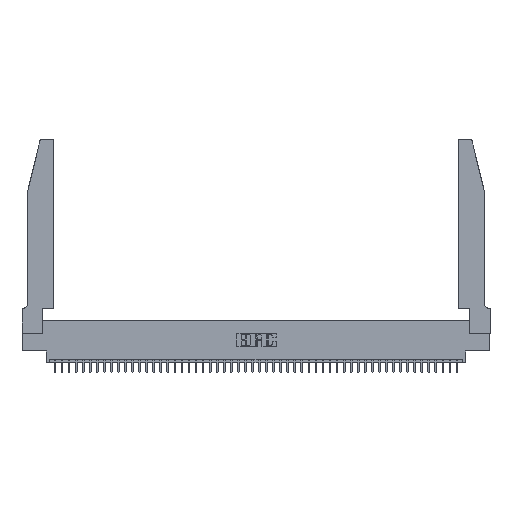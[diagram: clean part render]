
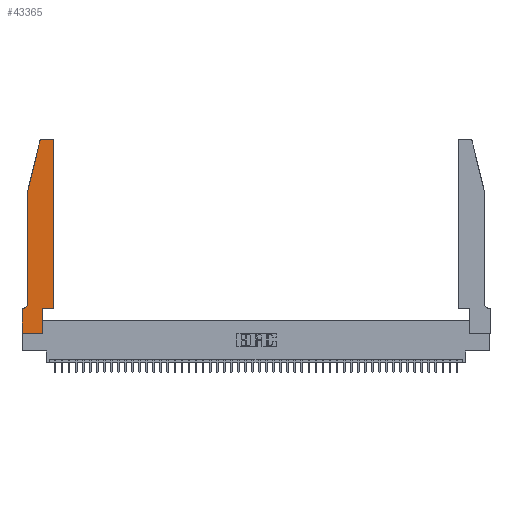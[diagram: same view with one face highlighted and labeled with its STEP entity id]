
A CAD part, top view. The second image highlights one B-rep face of the part: STEP entity #43365.
In plain terms, the highlighted planar face has unit normal (0, 0, 1).
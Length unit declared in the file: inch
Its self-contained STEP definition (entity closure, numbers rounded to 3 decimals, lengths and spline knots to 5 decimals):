
#545 = EDGE_CURVE ( 'NONE', #10601, #28192, #1196, .T. ) ;
#550 = VECTOR ( 'NONE', #3537, 39.37008 ) ;
#1196 = LINE ( 'NONE', #43739, #39708 ) ;
#1553 = VECTOR ( 'NONE', #6246, 39.37008 ) ;
#1555 = CARTESIAN_POINT ( 'NONE',  ( 0.2865, 0.35, 0.37 ) ) ;
#2090 = CARTESIAN_POINT ( 'NONE',  ( 0.2605, 2.75, 0.37 ) ) ;
#2269 = CIRCLE ( 'NONE', #10251, 0.03 ) ;
#2716 = AXIS2_PLACEMENT_3D ( 'NONE', #20783, #46829, #24542 ) ;
#2834 = CIRCLE ( 'NONE', #2716, 0.07 ) ;
#3537 = DIRECTION ( 'NONE',  ( 0., -1., 0. ) ) ;
#4672 = CARTESIAN_POINT ( 'NONE',  ( 0.0755, 0.35, 0.37 ) ) ;
#5462 = CARTESIAN_POINT ( 'NONE',  ( 0.0055, 0.35, 0.37 ) ) ;
#6246 = DIRECTION ( 'NONE',  ( 1., 0., 0. ) ) ;
#6683 = DIRECTION ( 'NONE',  ( 0., 0., 1. ) ) ;
#7171 = VECTOR ( 'NONE', #11006, 39.37008 ) ;
#8366 = VECTOR ( 'NONE', #9087, 39.37008 ) ;
#8771 = CARTESIAN_POINT ( 'NONE',  ( 0., 0.35, 0.37 ) ) ;
#8933 = CARTESIAN_POINT ( 'NONE',  ( 0.4505, 0.35, 0.37 ) ) ;
#9087 = DIRECTION ( 'NONE',  ( 0., 1., 0. ) ) ;
#9230 = VECTOR ( 'NONE', #24424, 39.37008 ) ;
#10251 = AXIS2_PLACEMENT_3D ( 'NONE', #28985, #6683, #32735 ) ;
#10310 = ORIENTED_EDGE ( 'NONE', *, *, #35866, .T. ) ;
#10337 = EDGE_LOOP ( 'NONE', ( #19519, #45235, #38002, #11027, #36350, #38988, #10310, #10574, #17658, #32203, #12888, #32692 ) ) ;
#10574 = ORIENTED_EDGE ( 'NONE', *, *, #18602, .T. ) ;
#10601 = VERTEX_POINT ( 'NONE', #22749 ) ;
#10939 = EDGE_CURVE ( 'NONE', #19008, #40300, #19494, .T. ) ;
#11006 = DIRECTION ( 'NONE',  ( 0., 1., 0. ) ) ;
#11027 = ORIENTED_EDGE ( 'NONE', *, *, #545, .T. ) ;
#12274 = CARTESIAN_POINT ( 'NONE',  ( 0.4505, 2.72, 0.37 ) ) ;
#12522 = DIRECTION ( 'NONE',  ( 1., 0., 0. ) ) ;
#12567 = EDGE_CURVE ( 'NONE', #17947, #24083, #40912, .T. ) ;
#12620 = LINE ( 'NONE', #20073, #31216 ) ;
#12888 = ORIENTED_EDGE ( 'NONE', *, *, #21205, .T. ) ;
#13624 = DIRECTION ( 'NONE',  ( 0., 0., 1. ) ) ;
#14572 = EDGE_CURVE ( 'NONE', #28192, #17947, #2834, .T. ) ;
#14744 = CARTESIAN_POINT ( 'NONE',  ( 0.4505, 0.35, 0.37 ) ) ;
#14824 = CARTESIAN_POINT ( 'NONE',  ( 0.4505, 0.35, 0.37 ) ) ;
#15294 = VERTEX_POINT ( 'NONE', #36340 ) ;
#15814 = EDGE_CURVE ( 'NONE', #40300, #15294, #27862, .T. ) ;
#15906 = DIRECTION ( 'NONE',  ( -1., 0., 0. ) ) ;
#16065 = PLANE ( 'NONE',  #46668 ) ;
#16336 = DIRECTION ( 'NONE',  ( -0.239, -0.971, 0. ) ) ;
#16352 = CARTESIAN_POINT ( 'NONE',  ( 0., 0.35, 0.37 ) ) ;
#17658 = ORIENTED_EDGE ( 'NONE', *, *, #23545, .T. ) ;
#17896 = AXIS2_PLACEMENT_3D ( 'NONE', #35896, #13624, #39667 ) ;
#17947 = VERTEX_POINT ( 'NONE', #5462 ) ;
#18275 = VERTEX_POINT ( 'NONE', #36865 ) ;
#18602 = EDGE_CURVE ( 'NONE', #41317, #45612, #21394, .T. ) ;
#19008 = VERTEX_POINT ( 'NONE', #12274 ) ;
#19279 = CARTESIAN_POINT ( 'NONE',  ( 0.25487, 2.72718, 0.37 ) ) ;
#19494 = CIRCLE ( 'NONE', #17896, 0.03 ) ;
#19519 = ORIENTED_EDGE ( 'NONE', *, *, #15814, .T. ) ;
#20073 = CARTESIAN_POINT ( 'NONE',  ( 0.0755, 2., 0.37 ) ) ;
#20783 = CARTESIAN_POINT ( 'NONE',  ( 0.0055, 0.42, 0.37 ) ) ;
#21067 = CARTESIAN_POINT ( 'NONE',  ( 0., 0., 0.37 ) ) ;
#21205 = EDGE_CURVE ( 'NONE', #40108, #19008, #36853, .T. ) ;
#21394 = LINE ( 'NONE', #21067, #1553 ) ;
#22749 = CARTESIAN_POINT ( 'NONE',  ( 0.0755, 2., 0.37 ) ) ;
#23545 = EDGE_CURVE ( 'NONE', #45612, #18275, #38035, .T. ) ;
#24083 = VERTEX_POINT ( 'NONE', #16352 ) ;
#24424 = DIRECTION ( 'NONE',  ( -1., 0., 0. ) ) ;
#24542 = DIRECTION ( 'NONE',  ( -1., 0., 0. ) ) ;
#24595 = LINE ( 'NONE', #14824, #43219 ) ;
#25198 = DIRECTION ( 'NONE',  ( 0., -1., 0. ) ) ;
#25268 = FACE_OUTER_BOUND ( 'NONE', #10337, .T. ) ;
#25862 = CARTESIAN_POINT ( 'NONE',  ( 0., 0., 0.37 ) ) ;
#27304 = EDGE_CURVE ( 'NONE', #29977, #10601, #12620, .T. ) ;
#27862 = LINE ( 'NONE', #2090, #9230 ) ;
#28192 = VERTEX_POINT ( 'NONE', #28501 ) ;
#28434 = CARTESIAN_POINT ( 'NONE',  ( 0.4205, 2.75, 0.37 ) ) ;
#28501 = CARTESIAN_POINT ( 'NONE',  ( 0.0755, 0.42, 0.37 ) ) ;
#28692 = VECTOR ( 'NONE', #15906, 39.37008 ) ;
#28985 = CARTESIAN_POINT ( 'NONE',  ( 0.284, 2.72, 0.37 ) ) ;
#29136 = EDGE_CURVE ( 'NONE', #18275, #40108, #24595, .T. ) ;
#29977 = VERTEX_POINT ( 'NONE', #19279 ) ;
#30090 = DIRECTION ( 'NONE',  ( 1., 0., 0. ) ) ;
#31216 = VECTOR ( 'NONE', #16336, 39.37008 ) ;
#32203 = ORIENTED_EDGE ( 'NONE', *, *, #29136, .T. ) ;
#32692 = ORIENTED_EDGE ( 'NONE', *, *, #10939, .T. ) ;
#32735 = DIRECTION ( 'NONE',  ( 1., 0., 0. ) ) ;
#34307 = CARTESIAN_POINT ( 'NONE',  ( 0., 0., 0.37 ) ) ;
#34788 = DIRECTION ( 'NONE',  ( 0., 0., 1. ) ) ;
#35866 = EDGE_CURVE ( 'NONE', #24083, #41317, #39055, .T. ) ;
#35896 = CARTESIAN_POINT ( 'NONE',  ( 0.4205, 2.72, 0.37 ) ) ;
#36340 = CARTESIAN_POINT ( 'NONE',  ( 0.284, 2.75, 0.37 ) ) ;
#36350 = ORIENTED_EDGE ( 'NONE', *, *, #14572, .T. ) ;
#36853 = LINE ( 'NONE', #14744, #7171 ) ;
#36865 = CARTESIAN_POINT ( 'NONE',  ( 0.2865, 0.35, 0.37 ) ) ;
#38002 = ORIENTED_EDGE ( 'NONE', *, *, #27304, .T. ) ;
#38035 = LINE ( 'NONE', #1555, #8366 ) ;
#38988 = ORIENTED_EDGE ( 'NONE', *, *, #12567, .T. ) ;
#39055 = LINE ( 'NONE', #25862, #550 ) ;
#39667 = DIRECTION ( 'NONE',  ( 1., 0., 0. ) ) ;
#39708 = VECTOR ( 'NONE', #25198, 39.37008 ) ;
#40108 = VERTEX_POINT ( 'NONE', #8933 ) ;
#40300 = VERTEX_POINT ( 'NONE', #28434 ) ;
#40912 = LINE ( 'NONE', #4672, #28692 ) ;
#41317 = VERTEX_POINT ( 'NONE', #34307 ) ;
#43219 = VECTOR ( 'NONE', #30090, 39.37008 ) ;
#43365 = ADVANCED_FACE ( 'NONE', ( #25268 ), #16065, .T. ) ;
#43739 = CARTESIAN_POINT ( 'NONE',  ( 0.0755, 2., 0.37 ) ) ;
#45235 = ORIENTED_EDGE ( 'NONE', *, *, #45628, .T. ) ;
#45612 = VERTEX_POINT ( 'NONE', #47359 ) ;
#45628 = EDGE_CURVE ( 'NONE', #15294, #29977, #2269, .T. ) ;
#46668 = AXIS2_PLACEMENT_3D ( 'NONE', #8771, #34788, #12522 ) ;
#46829 = DIRECTION ( 'NONE',  ( 0., 0., -1. ) ) ;
#47359 = CARTESIAN_POINT ( 'NONE',  ( 0.2865, 0., 0.37 ) ) ;
